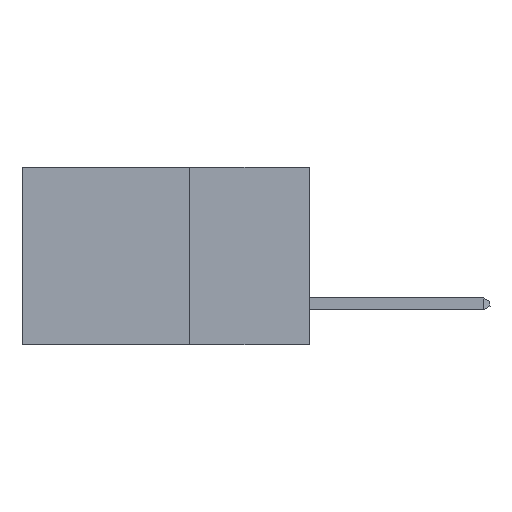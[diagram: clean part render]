
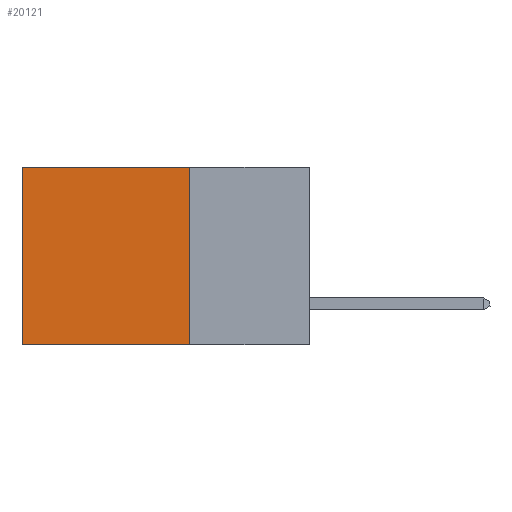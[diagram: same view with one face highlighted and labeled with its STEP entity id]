
A CAD part, left-side view. The second image highlights one B-rep face of the part: STEP entity #20121.
In plain terms, the highlighted planar face has unit normal (-1, 0, 0).
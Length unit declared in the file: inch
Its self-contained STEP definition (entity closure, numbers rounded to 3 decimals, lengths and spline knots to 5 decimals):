
#249 = CARTESIAN_POINT ( 'NONE',  ( 0.2875, 0.25, 0. ) ) ;
#315 = VERTEX_POINT ( 'NONE', #17650 ) ;
#1264 = VERTEX_POINT ( 'NONE', #18385 ) ;
#1407 = AXIS2_PLACEMENT_3D ( 'NONE', #5266, #17924, #7119 ) ;
#2024 = LINE ( 'NONE', #249, #16578 ) ;
#2072 = DIRECTION ( 'NONE',  ( 0., 1., 0. ) ) ;
#3068 = DIRECTION ( 'NONE',  ( 0., 0., -1. ) ) ;
#5266 = CARTESIAN_POINT ( 'NONE',  ( 0.2875, 0.25, 0. ) ) ;
#6045 = DIRECTION ( 'NONE',  ( 0., 1., 0. ) ) ;
#7119 = DIRECTION ( 'NONE',  ( 0., 0., -1. ) ) ;
#7884 = VECTOR ( 'NONE', #6045, 39.37008 ) ;
#9294 = CARTESIAN_POINT ( 'NONE',  ( 0.2875, 0.25, 0. ) ) ;
#9858 = VERTEX_POINT ( 'NONE', #10920 ) ;
#10920 = CARTESIAN_POINT ( 'NONE',  ( 0.2875, 0.6, 0. ) ) ;
#11876 = ORIENTED_EDGE ( 'NONE', *, *, #13978, .T. ) ;
#12734 = LINE ( 'NONE', #20430, #7884 ) ;
#12984 = EDGE_CURVE ( 'NONE', #9858, #315, #22023, .T. ) ;
#13216 = DIRECTION ( 'NONE',  ( 0., 0., -1. ) ) ;
#13726 = ORIENTED_EDGE ( 'NONE', *, *, #19683, .F. ) ;
#13978 = EDGE_CURVE ( 'NONE', #15716, #9858, #12734, .T. ) ;
#15098 = ORIENTED_EDGE ( 'NONE', *, *, #12984, .T. ) ;
#15221 = EDGE_CURVE ( 'NONE', #1264, #315, #17955, .T. ) ;
#15556 = VECTOR ( 'NONE', #3068, 39.37008 ) ;
#15716 = VERTEX_POINT ( 'NONE', #9294 ) ;
#16116 = PLANE ( 'NONE',  #1407 ) ;
#16255 = VECTOR ( 'NONE', #2072, 39.37008 ) ;
#16505 = ORIENTED_EDGE ( 'NONE', *, *, #15221, .F. ) ;
#16578 = VECTOR ( 'NONE', #13216, 39.37008 ) ;
#17650 = CARTESIAN_POINT ( 'NONE',  ( 0.2875, 0.6, -0.37 ) ) ;
#17924 = DIRECTION ( 'NONE',  ( 1., 0., 0. ) ) ;
#17955 = LINE ( 'NONE', #18475, #16255 ) ;
#18385 = CARTESIAN_POINT ( 'NONE',  ( 0.2875, 0.25, -0.37 ) ) ;
#18475 = CARTESIAN_POINT ( 'NONE',  ( 0.2875, 0.25, -0.37 ) ) ;
#19416 = CARTESIAN_POINT ( 'NONE',  ( 0.2875, 0.6, 0. ) ) ;
#19683 = EDGE_CURVE ( 'NONE', #15716, #1264, #2024, .T. ) ;
#20121 = ADVANCED_FACE ( 'NONE', ( #22474 ), #16116, .F. ) ;
#20430 = CARTESIAN_POINT ( 'NONE',  ( 0.2875, 0.25, 0. ) ) ;
#22023 = LINE ( 'NONE', #19416, #15556 ) ;
#22396 = EDGE_LOOP ( 'NONE', ( #15098, #16505, #13726, #11876 ) ) ;
#22474 = FACE_OUTER_BOUND ( 'NONE', #22396, .T. ) ;
